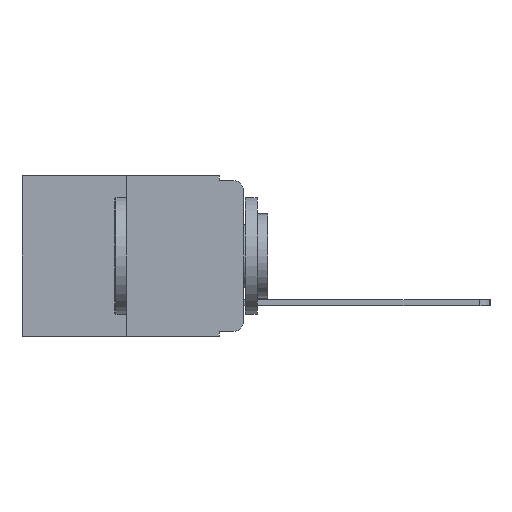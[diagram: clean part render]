
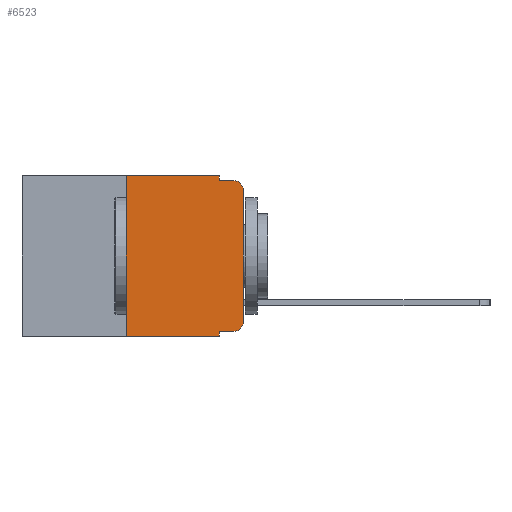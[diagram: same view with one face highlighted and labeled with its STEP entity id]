
A CAD part, left-side view. The second image highlights one B-rep face of the part: STEP entity #6523.
In plain terms, the highlighted planar face has unit normal (-1, 0, 0).
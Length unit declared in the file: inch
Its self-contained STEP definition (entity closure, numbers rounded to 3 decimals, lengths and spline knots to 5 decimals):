
#182 = VERTEX_POINT ( 'NONE', #6218 ) ;
#361 = CARTESIAN_POINT ( 'NONE',  ( 0., 0.02, -0.313 ) ) ;
#471 = LINE ( 'NONE', #12254, #4442 ) ;
#719 = EDGE_CURVE ( 'NONE', #182, #13393, #13621, .T. ) ;
#749 = DIRECTION ( 'NONE',  ( 0., 0., -1. ) ) ;
#847 = VERTEX_POINT ( 'NONE', #16020 ) ;
#1347 = ORIENTED_EDGE ( 'NONE', *, *, #17969, .T. ) ;
#2099 = DIRECTION ( 'NONE',  ( 0., 0., -1. ) ) ;
#2119 = CARTESIAN_POINT ( 'NONE',  ( 0., 0.051, -0.01 ) ) ;
#2309 = CARTESIAN_POINT ( 'NONE',  ( 0., 0.473, -0.343 ) ) ;
#2329 = EDGE_CURVE ( 'NONE', #15364, #6452, #15068, .T. ) ;
#2387 = FACE_OUTER_BOUND ( 'NONE', #16872, .T. ) ;
#2837 = VECTOR ( 'NONE', #15166, 39.37008 ) ;
#2878 = VECTOR ( 'NONE', #14378, 39.37008 ) ;
#3803 = CIRCLE ( 'NONE', #6344, 0.02 ) ;
#3929 = LINE ( 'NONE', #15788, #2878 ) ;
#4097 = CARTESIAN_POINT ( 'NONE',  ( 0., 0.473, 0. ) ) ;
#4159 = ORIENTED_EDGE ( 'NONE', *, *, #11447, .F. ) ;
#4304 = CARTESIAN_POINT ( 'NONE',  ( 0., 0.25, 0. ) ) ;
#4442 = VECTOR ( 'NONE', #6505, 39.37008 ) ;
#4511 = EDGE_CURVE ( 'NONE', #10058, #182, #3803, .T. ) ;
#4753 = CARTESIAN_POINT ( 'NONE',  ( 0., 0.25, 0. ) ) ;
#4928 = VERTEX_POINT ( 'NONE', #14874 ) ;
#5948 = VECTOR ( 'NONE', #14224, 39.37008 ) ;
#6007 = VECTOR ( 'NONE', #17254, 39.37008 ) ;
#6215 = CARTESIAN_POINT ( 'NONE',  ( 0., 0.02, -0.333 ) ) ;
#6218 = CARTESIAN_POINT ( 'NONE',  ( 0., 0., -0.313 ) ) ;
#6344 = AXIS2_PLACEMENT_3D ( 'NONE', #361, #11223, #2099 ) ;
#6422 = ORIENTED_EDGE ( 'NONE', *, *, #719, .T. ) ;
#6452 = VERTEX_POINT ( 'NONE', #14174 ) ;
#6505 = DIRECTION ( 'NONE',  ( 0., 0., -1. ) ) ;
#6521 = ORIENTED_EDGE ( 'NONE', *, *, #2329, .F. ) ;
#6523 = ADVANCED_FACE ( 'NONE', ( #2387 ), #15696, .F. ) ;
#6873 = AXIS2_PLACEMENT_3D ( 'NONE', #9335, #19154, #10778 ) ;
#6889 = VECTOR ( 'NONE', #8452, 39.37008 ) ;
#7015 = LINE ( 'NONE', #13783, #2837 ) ;
#7219 = ORIENTED_EDGE ( 'NONE', *, *, #16139, .F. ) ;
#8452 = DIRECTION ( 'NONE',  ( 0., 0., 1. ) ) ;
#8513 = ORIENTED_EDGE ( 'NONE', *, *, #17052, .F. ) ;
#8872 = VECTOR ( 'NONE', #12683, 39.37008 ) ;
#8894 = VECTOR ( 'NONE', #17350, 39.37008 ) ;
#9335 = CARTESIAN_POINT ( 'NONE',  ( 0., 0.02, -0.03 ) ) ;
#9413 = CARTESIAN_POINT ( 'NONE',  ( 0., 0.051, -0.01 ) ) ;
#10000 = ORIENTED_EDGE ( 'NONE', *, *, #10479, .T. ) ;
#10058 = VERTEX_POINT ( 'NONE', #6215 ) ;
#10085 = DIRECTION ( 'NONE',  ( 1., 0., 0. ) ) ;
#10479 = EDGE_CURVE ( 'NONE', #4928, #10058, #3929, .T. ) ;
#10627 = CIRCLE ( 'NONE', #6873, 0.02 ) ;
#10637 = AXIS2_PLACEMENT_3D ( 'NONE', #4097, #10085, #749 ) ;
#10778 = DIRECTION ( 'NONE',  ( 0., 0., -1. ) ) ;
#11223 = DIRECTION ( 'NONE',  ( -1., 0., 0. ) ) ;
#11447 = EDGE_CURVE ( 'NONE', #4928, #847, #7015, .T. ) ;
#12080 = VERTEX_POINT ( 'NONE', #17933 ) ;
#12254 = CARTESIAN_POINT ( 'NONE',  ( 0., 0.051, 0. ) ) ;
#12383 = EDGE_CURVE ( 'NONE', #13236, #15364, #13702, .T. ) ;
#12683 = DIRECTION ( 'NONE',  ( 0., -1., 0. ) ) ;
#13096 = ORIENTED_EDGE ( 'NONE', *, *, #15686, .T. ) ;
#13236 = VERTEX_POINT ( 'NONE', #18807 ) ;
#13393 = VERTEX_POINT ( 'NONE', #13536 ) ;
#13475 = VERTEX_POINT ( 'NONE', #9413 ) ;
#13536 = CARTESIAN_POINT ( 'NONE',  ( 0., 0., -0.03 ) ) ;
#13543 = CARTESIAN_POINT ( 'NONE',  ( 0., 0., 0. ) ) ;
#13621 = LINE ( 'NONE', #13543, #6889 ) ;
#13702 = LINE ( 'NONE', #4304, #6007 ) ;
#13783 = CARTESIAN_POINT ( 'NONE',  ( 0., 0.051, 0. ) ) ;
#14174 = CARTESIAN_POINT ( 'NONE',  ( 0., 0.051, 0. ) ) ;
#14224 = DIRECTION ( 'NONE',  ( 0., -1., 0. ) ) ;
#14378 = DIRECTION ( 'NONE',  ( 0., -1., 0. ) ) ;
#14874 = CARTESIAN_POINT ( 'NONE',  ( 0., 0.051, -0.333 ) ) ;
#15068 = LINE ( 'NONE', #16334, #8894 ) ;
#15166 = DIRECTION ( 'NONE',  ( 0., 0., -1. ) ) ;
#15364 = VERTEX_POINT ( 'NONE', #4753 ) ;
#15686 = EDGE_CURVE ( 'NONE', #13236, #847, #16891, .T. ) ;
#15696 = PLANE ( 'NONE',  #10637 ) ;
#15788 = CARTESIAN_POINT ( 'NONE',  ( 0., 0.051, -0.333 ) ) ;
#16020 = CARTESIAN_POINT ( 'NONE',  ( 0., 0.051, -0.343 ) ) ;
#16139 = EDGE_CURVE ( 'NONE', #6452, #13475, #471, .T. ) ;
#16334 = CARTESIAN_POINT ( 'NONE',  ( 0., 0.473, 0. ) ) ;
#16816 = LINE ( 'NONE', #2119, #8872 ) ;
#16872 = EDGE_LOOP ( 'NONE', ( #6422, #1347, #8513, #7219, #6521, #17846, #13096, #4159, #10000, #17483 ) ) ;
#16891 = LINE ( 'NONE', #2309, #5948 ) ;
#17052 = EDGE_CURVE ( 'NONE', #13475, #12080, #16816, .T. ) ;
#17254 = DIRECTION ( 'NONE',  ( 0., 0., 1. ) ) ;
#17350 = DIRECTION ( 'NONE',  ( 0., -1., 0. ) ) ;
#17483 = ORIENTED_EDGE ( 'NONE', *, *, #4511, .T. ) ;
#17846 = ORIENTED_EDGE ( 'NONE', *, *, #12383, .F. ) ;
#17933 = CARTESIAN_POINT ( 'NONE',  ( 0., 0.02, -0.01 ) ) ;
#17969 = EDGE_CURVE ( 'NONE', #13393, #12080, #10627, .T. ) ;
#18807 = CARTESIAN_POINT ( 'NONE',  ( 0., 0.25, -0.343 ) ) ;
#19154 = DIRECTION ( 'NONE',  ( -1., 0., 0. ) ) ;
